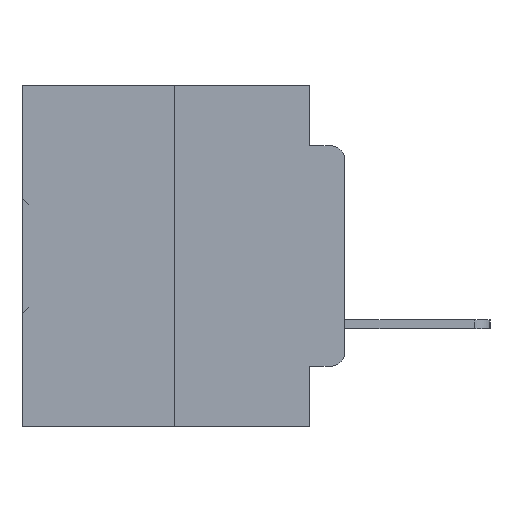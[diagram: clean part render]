
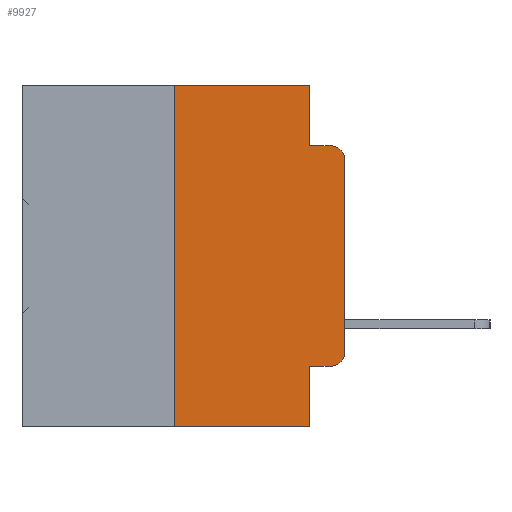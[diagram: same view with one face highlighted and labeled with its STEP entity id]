
A CAD part, left-side view. The second image highlights one B-rep face of the part: STEP entity #9927.
In plain terms, the highlighted planar face has unit normal (-1, 0, 0).
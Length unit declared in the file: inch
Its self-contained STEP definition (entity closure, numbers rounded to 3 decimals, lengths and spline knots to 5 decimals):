
#124 = VERTEX_POINT ( 'NONE', #26783 ) ;
#971 = CARTESIAN_POINT ( 'NONE',  ( 0., 0.051, -0.5 ) ) ;
#1321 = ORIENTED_EDGE ( 'NONE', *, *, #4843, .T. ) ;
#2322 = CARTESIAN_POINT ( 'NONE',  ( 0., 0.051, 0. ) ) ;
#3293 = DIRECTION ( 'NONE',  ( 1., 0., 0. ) ) ;
#3532 = LINE ( 'NONE', #8252, #9949 ) ;
#3563 = CIRCLE ( 'NONE', #6789, 0.02 ) ;
#3774 = LINE ( 'NONE', #15102, #17520 ) ;
#3938 = CARTESIAN_POINT ( 'NONE',  ( 0., 0.25, 0. ) ) ;
#4761 = ORIENTED_EDGE ( 'NONE', *, *, #10321, .F. ) ;
#4843 = EDGE_CURVE ( 'NONE', #34055, #11881, #5948, .T. ) ;
#4987 = ORIENTED_EDGE ( 'NONE', *, *, #27332, .T. ) ;
#5459 = ORIENTED_EDGE ( 'NONE', *, *, #6018, .F. ) ;
#5948 = CIRCLE ( 'NONE', #28754, 0.02 ) ;
#6012 = DIRECTION ( 'NONE',  ( -1., 0., 0. ) ) ;
#6018 = EDGE_CURVE ( 'NONE', #28743, #21825, #29251, .T. ) ;
#6301 = FACE_OUTER_BOUND ( 'NONE', #35167, .T. ) ;
#6412 = CARTESIAN_POINT ( 'NONE',  ( 0., 0.02, -0.1085 ) ) ;
#6704 = EDGE_CURVE ( 'NONE', #27099, #34055, #28788, .T. ) ;
#6789 = AXIS2_PLACEMENT_3D ( 'NONE', #6412, #25532, #9154 ) ;
#6811 = EDGE_CURVE ( 'NONE', #124, #26116, #3532, .T. ) ;
#6918 = ORIENTED_EDGE ( 'NONE', *, *, #10539, .F. ) ;
#7367 = ORIENTED_EDGE ( 'NONE', *, *, #32317, .F. ) ;
#7578 = VERTEX_POINT ( 'NONE', #30631 ) ;
#7784 = CARTESIAN_POINT ( 'NONE',  ( 0., 0.051, -0.4115 ) ) ;
#7836 = AXIS2_PLACEMENT_3D ( 'NONE', #19692, #3293, #22447 ) ;
#8252 = CARTESIAN_POINT ( 'NONE',  ( 0., 0.473, -0.5 ) ) ;
#9154 = DIRECTION ( 'NONE',  ( 0., 0., -1. ) ) ;
#9246 = DIRECTION ( 'NONE',  ( 0., -1., 0. ) ) ;
#9927 = ADVANCED_FACE ( 'NONE', ( #6301 ), #14207, .F. ) ;
#9949 = VECTOR ( 'NONE', #21889, 39.37008 ) ;
#10321 = EDGE_CURVE ( 'NONE', #27099, #26116, #28916, .T. ) ;
#10428 = DIRECTION ( 'NONE',  ( 0., 0., -1. ) ) ;
#10539 = EDGE_CURVE ( 'NONE', #32726, #28743, #20388, .T. ) ;
#11575 = ORIENTED_EDGE ( 'NONE', *, *, #20481, .T. ) ;
#11881 = VERTEX_POINT ( 'NONE', #15861 ) ;
#12359 = LINE ( 'NONE', #31967, #17979 ) ;
#13055 = DIRECTION ( 'NONE',  ( 0., 0., 1. ) ) ;
#13392 = VECTOR ( 'NONE', #29608, 39.37008 ) ;
#13679 = CARTESIAN_POINT ( 'NONE',  ( 0., 0.051, 0. ) ) ;
#13888 = VECTOR ( 'NONE', #34795, 39.37008 ) ;
#14207 = PLANE ( 'NONE',  #7836 ) ;
#15102 = CARTESIAN_POINT ( 'NONE',  ( 0., 0., 0. ) ) ;
#15861 = CARTESIAN_POINT ( 'NONE',  ( 0., 0., -0.3915 ) ) ;
#16270 = CARTESIAN_POINT ( 'NONE',  ( 0., 0.051, -0.4115 ) ) ;
#16788 = VERTEX_POINT ( 'NONE', #19957 ) ;
#17520 = VECTOR ( 'NONE', #17865, 39.37008 ) ;
#17865 = DIRECTION ( 'NONE',  ( 0., 0., 1. ) ) ;
#17979 = VECTOR ( 'NONE', #34706, 39.37008 ) ;
#18600 = CARTESIAN_POINT ( 'NONE',  ( 0., 0.25, 0. ) ) ;
#19692 = CARTESIAN_POINT ( 'NONE',  ( 0., 0.473, 0. ) ) ;
#19957 = CARTESIAN_POINT ( 'NONE',  ( 0., 0.02, -0.0885 ) ) ;
#20388 = LINE ( 'NONE', #25626, #34861 ) ;
#20481 = EDGE_CURVE ( 'NONE', #11881, #7578, #3774, .T. ) ;
#20819 = VECTOR ( 'NONE', #10428, 39.37008 ) ;
#21825 = VERTEX_POINT ( 'NONE', #34544 ) ;
#21889 = DIRECTION ( 'NONE',  ( 0., -1., 0. ) ) ;
#22397 = CARTESIAN_POINT ( 'NONE',  ( 0., 0.02, -0.3915 ) ) ;
#22447 = DIRECTION ( 'NONE',  ( 0., 0., -1. ) ) ;
#24740 = LINE ( 'NONE', #18600, #31119 ) ;
#25136 = DIRECTION ( 'NONE',  ( 0., 0., -1. ) ) ;
#25532 = DIRECTION ( 'NONE',  ( -1., 0., 0. ) ) ;
#25626 = CARTESIAN_POINT ( 'NONE',  ( 0., 0.473, 0. ) ) ;
#26116 = VERTEX_POINT ( 'NONE', #971 ) ;
#26783 = CARTESIAN_POINT ( 'NONE',  ( 0., 0.25, -0.5 ) ) ;
#27099 = VERTEX_POINT ( 'NONE', #16270 ) ;
#27332 = EDGE_CURVE ( 'NONE', #7578, #16788, #3563, .T. ) ;
#28290 = ORIENTED_EDGE ( 'NONE', *, *, #6811, .T. ) ;
#28743 = VERTEX_POINT ( 'NONE', #13679 ) ;
#28754 = AXIS2_PLACEMENT_3D ( 'NONE', #22397, #6012, #25136 ) ;
#28788 = LINE ( 'NONE', #7784, #13392 ) ;
#28916 = LINE ( 'NONE', #2322, #20819 ) ;
#29251 = LINE ( 'NONE', #32043, #13888 ) ;
#29608 = DIRECTION ( 'NONE',  ( 0., -1., 0. ) ) ;
#30631 = CARTESIAN_POINT ( 'NONE',  ( 0., 0., -0.1085 ) ) ;
#31119 = VECTOR ( 'NONE', #13055, 39.37008 ) ;
#31641 = EDGE_CURVE ( 'NONE', #21825, #16788, #12359, .T. ) ;
#31967 = CARTESIAN_POINT ( 'NONE',  ( 0., 0.051, -0.0885 ) ) ;
#32043 = CARTESIAN_POINT ( 'NONE',  ( 0., 0.051, 0. ) ) ;
#32317 = EDGE_CURVE ( 'NONE', #124, #32726, #24740, .T. ) ;
#32726 = VERTEX_POINT ( 'NONE', #3938 ) ;
#33817 = ORIENTED_EDGE ( 'NONE', *, *, #6704, .T. ) ;
#34055 = VERTEX_POINT ( 'NONE', #34674 ) ;
#34239 = ORIENTED_EDGE ( 'NONE', *, *, #31641, .F. ) ;
#34544 = CARTESIAN_POINT ( 'NONE',  ( 0., 0.051, -0.0885 ) ) ;
#34674 = CARTESIAN_POINT ( 'NONE',  ( 0., 0.02, -0.4115 ) ) ;
#34706 = DIRECTION ( 'NONE',  ( 0., -1., 0. ) ) ;
#34795 = DIRECTION ( 'NONE',  ( 0., 0., -1. ) ) ;
#34861 = VECTOR ( 'NONE', #9246, 39.37008 ) ;
#35167 = EDGE_LOOP ( 'NONE', ( #11575, #4987, #34239, #5459, #6918, #7367, #28290, #4761, #33817, #1321 ) ) ;
